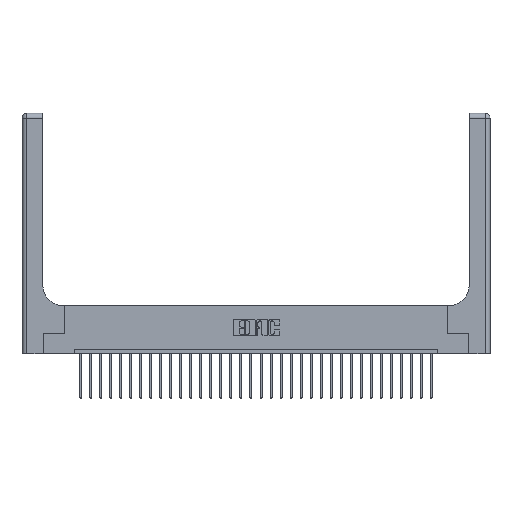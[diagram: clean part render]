
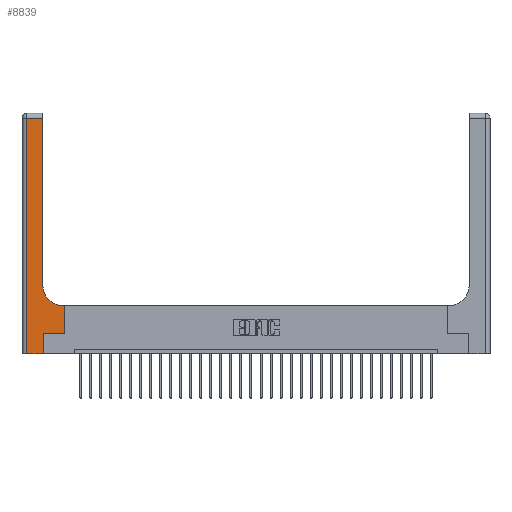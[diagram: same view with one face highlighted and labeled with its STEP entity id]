
A CAD part, top view. The second image highlights one B-rep face of the part: STEP entity #8839.
In plain terms, the highlighted planar face has unit normal (0, 0, 1).
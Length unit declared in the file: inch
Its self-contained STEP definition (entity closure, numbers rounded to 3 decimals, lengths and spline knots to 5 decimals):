
#330 = DIRECTION ( 'NONE',  ( 0., 0., -1. ) ) ;
#490 = EDGE_CURVE ( 'NONE', #3364, #25847, #23790, .T. ) ;
#990 = EDGE_CURVE ( 'NONE', #20452, #25909, #25370, .T. ) ;
#1594 = VERTEX_POINT ( 'NONE', #11545 ) ;
#1640 = CARTESIAN_POINT ( 'NONE',  ( 0., 0., 0.37 ) ) ;
#1767 = DIRECTION ( 'NONE',  ( 1., 0., 0. ) ) ;
#3190 = DIRECTION ( 'NONE',  ( 0., 1., 0. ) ) ;
#3364 = VERTEX_POINT ( 'NONE', #24861 ) ;
#3633 = LINE ( 'NONE', #14991, #16014 ) ;
#3887 = VECTOR ( 'NONE', #1767, 39.37008 ) ;
#4551 = AXIS2_PLACEMENT_3D ( 'NONE', #5981, #23777, #12222 ) ;
#4556 = PLANE ( 'NONE',  #26877 ) ;
#4842 = CARTESIAN_POINT ( 'NONE',  ( 0.26, 0.85, 0.37 ) ) ;
#4922 = ORIENTED_EDGE ( 'NONE', *, *, #27357, .T. ) ;
#5308 = VECTOR ( 'NONE', #3190, 39.37008 ) ;
#5387 = CARTESIAN_POINT ( 'NONE',  ( 0.26, 3., 0.37 ) ) ;
#5455 = LINE ( 'NONE', #7514, #9291 ) ;
#5981 = CARTESIAN_POINT ( 'NONE',  ( 0.51, 0.85, 0.37 ) ) ;
#6558 = EDGE_CURVE ( 'NONE', #10278, #3364, #13551, .T. ) ;
#6816 = ORIENTED_EDGE ( 'NONE', *, *, #18779, .T. ) ;
#7322 = CARTESIAN_POINT ( 'NONE',  ( 0.26, 0.6, 0.37 ) ) ;
#7508 = LINE ( 'NONE', #14470, #21788 ) ;
#7514 = CARTESIAN_POINT ( 'NONE',  ( 0.265, 0., 0.37 ) ) ;
#7760 = CARTESIAN_POINT ( 'NONE',  ( 0.51, 0.6, 0.37 ) ) ;
#8734 = EDGE_CURVE ( 'NONE', #25909, #10278, #7508, .T. ) ;
#8839 = ADVANCED_FACE ( 'NONE', ( #16066 ), #4556, .F. ) ;
#9071 = DIRECTION ( 'NONE',  ( -1., 0., 0. ) ) ;
#9291 = VECTOR ( 'NONE', #14192, 39.37008 ) ;
#9421 = CARTESIAN_POINT ( 'NONE',  ( 0.265, 0., 0.37 ) ) ;
#9802 = DIRECTION ( 'NONE',  ( -1., 0., 0. ) ) ;
#10278 = VERTEX_POINT ( 'NONE', #14245 ) ;
#10866 = CARTESIAN_POINT ( 'NONE',  ( 0.265, 0.25, 0.37 ) ) ;
#10950 = CARTESIAN_POINT ( 'NONE',  ( 0.06, 3., 0.37 ) ) ;
#11545 = CARTESIAN_POINT ( 'NONE',  ( 0.528, 0.25, 0.37 ) ) ;
#11819 = DIRECTION ( 'NONE',  ( -1., 0., 0. ) ) ;
#12222 = DIRECTION ( 'NONE',  ( 1., 0., 0. ) ) ;
#12862 = VERTEX_POINT ( 'NONE', #7760 ) ;
#13551 = LINE ( 'NONE', #10950, #26205 ) ;
#13699 = CARTESIAN_POINT ( 'NONE',  ( 0., 3., 0.37 ) ) ;
#14192 = DIRECTION ( 'NONE',  ( 0., 1., 0. ) ) ;
#14245 = CARTESIAN_POINT ( 'NONE',  ( 0.06, 2.94, 0.37 ) ) ;
#14293 = CIRCLE ( 'NONE', #4551, 0.25 ) ;
#14470 = CARTESIAN_POINT ( 'NONE',  ( 0., 2.94, 0.37 ) ) ;
#14942 = CARTESIAN_POINT ( 'NONE',  ( 0.26, 2.94, 0.37 ) ) ;
#14991 = CARTESIAN_POINT ( 'NONE',  ( 0.528, 0.25, 0.37 ) ) ;
#15545 = LINE ( 'NONE', #10866, #18541 ) ;
#15627 = ORIENTED_EDGE ( 'NONE', *, *, #21021, .T. ) ;
#16014 = VECTOR ( 'NONE', #16921, 39.37008 ) ;
#16066 = FACE_OUTER_BOUND ( 'NONE', #28265, .T. ) ;
#16786 = ORIENTED_EDGE ( 'NONE', *, *, #990, .T. ) ;
#16921 = DIRECTION ( 'NONE',  ( 0., 1., 0. ) ) ;
#17558 = ORIENTED_EDGE ( 'NONE', *, *, #21185, .T. ) ;
#18377 = EDGE_CURVE ( 'NONE', #12862, #20452, #14293, .T. ) ;
#18541 = VECTOR ( 'NONE', #25665, 39.37008 ) ;
#18779 = EDGE_CURVE ( 'NONE', #21992, #1594, #15545, .T. ) ;
#19855 = DIRECTION ( 'NONE',  ( 0., -1., 0. ) ) ;
#20015 = VECTOR ( 'NONE', #11819, 39.37008 ) ;
#20452 = VERTEX_POINT ( 'NONE', #4842 ) ;
#21021 = EDGE_CURVE ( 'NONE', #25847, #21992, #5455, .T. ) ;
#21185 = EDGE_CURVE ( 'NONE', #25074, #12862, #23087, .T. ) ;
#21788 = VECTOR ( 'NONE', #9802, 39.37008 ) ;
#21796 = ORIENTED_EDGE ( 'NONE', *, *, #6558, .T. ) ;
#21992 = VERTEX_POINT ( 'NONE', #26697 ) ;
#22167 = ORIENTED_EDGE ( 'NONE', *, *, #490, .T. ) ;
#22431 = ORIENTED_EDGE ( 'NONE', *, *, #18377, .T. ) ;
#23087 = LINE ( 'NONE', #7322, #20015 ) ;
#23629 = ORIENTED_EDGE ( 'NONE', *, *, #8734, .T. ) ;
#23777 = DIRECTION ( 'NONE',  ( 0., 0., -1. ) ) ;
#23790 = LINE ( 'NONE', #1640, #3887 ) ;
#24594 = CARTESIAN_POINT ( 'NONE',  ( 0.528, 0.6, 0.37 ) ) ;
#24861 = CARTESIAN_POINT ( 'NONE',  ( 0.06, 0., 0.37 ) ) ;
#25074 = VERTEX_POINT ( 'NONE', #24594 ) ;
#25370 = LINE ( 'NONE', #5387, #5308 ) ;
#25665 = DIRECTION ( 'NONE',  ( 1., 0., 0. ) ) ;
#25847 = VERTEX_POINT ( 'NONE', #9421 ) ;
#25909 = VERTEX_POINT ( 'NONE', #14942 ) ;
#26205 = VECTOR ( 'NONE', #19855, 39.37008 ) ;
#26697 = CARTESIAN_POINT ( 'NONE',  ( 0.265, 0.25, 0.37 ) ) ;
#26877 = AXIS2_PLACEMENT_3D ( 'NONE', #13699, #330, #9071 ) ;
#27357 = EDGE_CURVE ( 'NONE', #1594, #25074, #3633, .T. ) ;
#28265 = EDGE_LOOP ( 'NONE', ( #16786, #23629, #21796, #22167, #15627, #6816, #4922, #17558, #22431 ) ) ;
